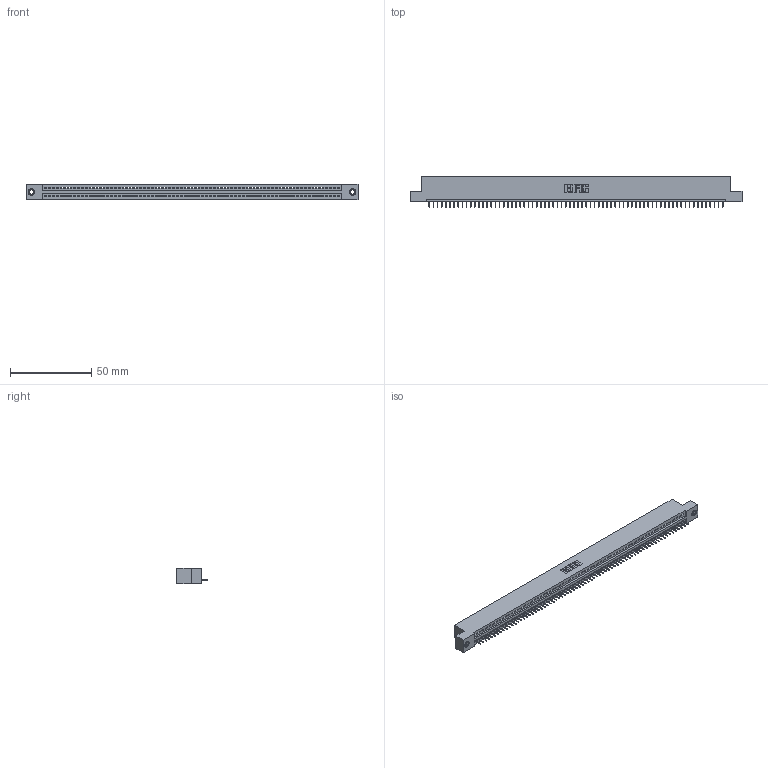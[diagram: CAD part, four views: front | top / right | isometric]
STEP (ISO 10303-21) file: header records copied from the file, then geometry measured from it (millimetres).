
FILE_DESCRIPTION (( 'STEP AP203' ), '1' );
FILE_NAME ('395-072-525-107.STEP', '2020-09-25T07:07:16', ( '' ), ( '' ), 'SwSTEP 2.0', 'SolidWorks 2020', '' );
FILE_SCHEMA (( 'CONFIG_CONTROL_DESIGN' ));
Length unit declared in the file: inch
Products named in the file (4): 395-072-525-107; 345-292-001_345-293-125; 345-250-001_345-250-005-103; 345 Part_Flush Mounting Lugs - 0.156 Dia-TI
Assembly tree (75 placements, depth 2):
  395-072-525-107
    345 Part_Flush Mounting Lugs - 0.156 Dia-TI
    345-292-001_345-293-125  x72
    345-250-001_345-250-005-103  x2
Bounding box: 204.09 x 18.72 x 9.4 mm (x, y, z)
Volume: 19322.8 mm3; surface area: 25138.3 mm2
Topology: 75 solids, 75 shells, 4650 faces, 13437 edges, 8662 vertices
Faces by surface type: plane 3424, cylinder 1210, cone 12, torus 4
Entity records: 51410 total; most frequent: CARTESIAN_POINT 8883, ORIENTED_EDGE 8882, DIRECTION 7743, EDGE_CURVE 4441, VECTOR 4005, LINE 4005, VERTEX_POINT 2952, AXIS2_PLACEMENT_3D 1869
